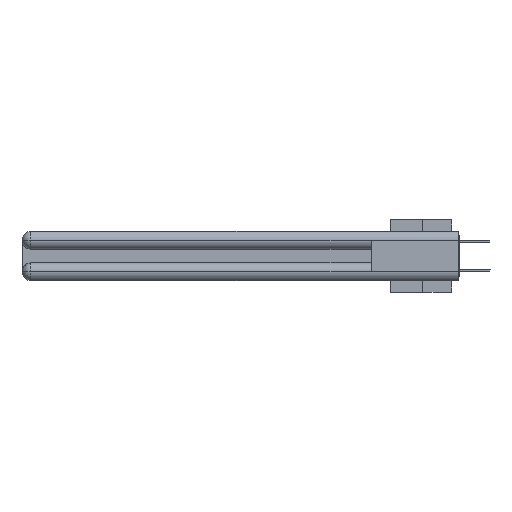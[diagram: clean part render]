
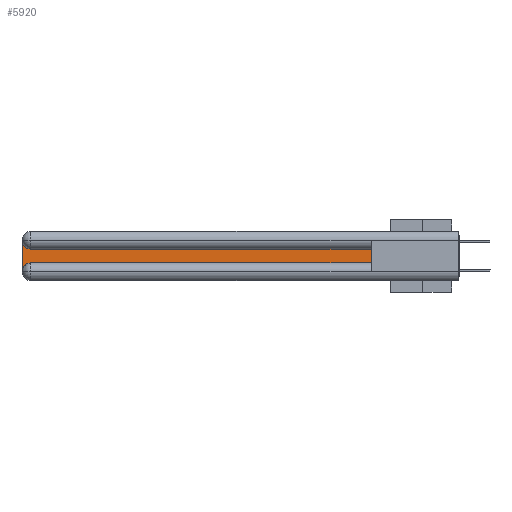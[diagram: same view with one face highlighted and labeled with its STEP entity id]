
A CAD part, left-side view. The second image highlights one B-rep face of the part: STEP entity #5920.
In plain terms, the highlighted planar face has unit normal (-1, 0, 0).
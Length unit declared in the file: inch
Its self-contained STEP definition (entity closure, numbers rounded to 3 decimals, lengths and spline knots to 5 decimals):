
#1481 = CARTESIAN_POINT ( 'NONE',  ( 0.075, 0.6, -0.2175 ) ) ;
#1792 = CARTESIAN_POINT ( 'NONE',  ( 0.075, 0.6, -0.2175 ) ) ;
#2102 = ORIENTED_EDGE ( 'NONE', *, *, #15685, .T. ) ;
#2731 = ORIENTED_EDGE ( 'NONE', *, *, #14628, .T. ) ;
#2751 = ORIENTED_EDGE ( 'NONE', *, *, #28958, .T. ) ;
#3888 = CARTESIAN_POINT ( 'NONE',  ( 0.075, 3., -0.2775 ) ) ;
#4295 = DIRECTION ( 'NONE',  ( 0., 0., 1. ) ) ;
#4319 = LINE ( 'NONE', #1481, #8653 ) ;
#4943 = CARTESIAN_POINT ( 'NONE',  ( 0.075, 2.94, -0.1225 ) ) ;
#5920 = ADVANCED_FACE ( 'NONE', ( #34883 ), #7283, .F. ) ;
#6153 = LINE ( 'NONE', #12125, #27566 ) ;
#7283 = PLANE ( 'NONE',  #14987 ) ;
#7659 = ORIENTED_EDGE ( 'NONE', *, *, #33788, .T. ) ;
#8567 = LINE ( 'NONE', #12396, #33830 ) ;
#8653 = VECTOR ( 'NONE', #4295, 39.37008 ) ;
#9470 = DIRECTION ( 'NONE',  ( 1., 0., 0. ) ) ;
#9493 = LINE ( 'NONE', #20822, #21748 ) ;
#10178 = DIRECTION ( 'NONE',  ( 0., -1., 0. ) ) ;
#11277 = ORIENTED_EDGE ( 'NONE', *, *, #23849, .T. ) ;
#11372 = EDGE_CURVE ( 'NONE', #14433, #11629, #6153, .T. ) ;
#11629 = VERTEX_POINT ( 'NONE', #3888 ) ;
#12125 = CARTESIAN_POINT ( 'NONE',  ( 0.075, 3., -0.2175 ) ) ;
#12335 = CARTESIAN_POINT ( 'NONE',  ( 0.075, 3., -0.0625 ) ) ;
#12396 = CARTESIAN_POINT ( 'NONE',  ( 0.075, 0.6, -0.1225 ) ) ;
#14433 = VERTEX_POINT ( 'NONE', #12335 ) ;
#14442 = VERTEX_POINT ( 'NONE', #32348 ) ;
#14628 = EDGE_CURVE ( 'NONE', #14442, #19472, #8567, .T. ) ;
#14987 = AXIS2_PLACEMENT_3D ( 'NONE', #15819, #24259, #35648 ) ;
#15364 = AXIS2_PLACEMENT_3D ( 'NONE', #23409, #9470, #26465 ) ;
#15685 = EDGE_CURVE ( 'NONE', #11629, #19381, #32975, .T. ) ;
#15819 = CARTESIAN_POINT ( 'NONE',  ( 0.075, 3., -0.1225 ) ) ;
#15835 = VERTEX_POINT ( 'NONE', #1792 ) ;
#16766 = CARTESIAN_POINT ( 'NONE',  ( 0.075, 2.94, -0.0625 ) ) ;
#17237 = DIRECTION ( 'NONE',  ( 1., 0., 0. ) ) ;
#19381 = VERTEX_POINT ( 'NONE', #26808 ) ;
#19472 = VERTEX_POINT ( 'NONE', #4943 ) ;
#19587 = DIRECTION ( 'NONE',  ( 0., 0., -1. ) ) ;
#20557 = DIRECTION ( 'NONE',  ( 0., 0., -1. ) ) ;
#20822 = CARTESIAN_POINT ( 'NONE',  ( 0.075, 0.6, -0.2175 ) ) ;
#21748 = VECTOR ( 'NONE', #10178, 39.37008 ) ;
#23409 = CARTESIAN_POINT ( 'NONE',  ( 0.075, 2.94, -0.2775 ) ) ;
#23521 = CIRCLE ( 'NONE', #31676, 0.06 ) ;
#23849 = EDGE_CURVE ( 'NONE', #19381, #15835, #9493, .T. ) ;
#24007 = DIRECTION ( 'NONE',  ( 0., 1., 0. ) ) ;
#24259 = DIRECTION ( 'NONE',  ( 1., 0., 0. ) ) ;
#24705 = ORIENTED_EDGE ( 'NONE', *, *, #11372, .T. ) ;
#26465 = DIRECTION ( 'NONE',  ( 0., 0., -1. ) ) ;
#26808 = CARTESIAN_POINT ( 'NONE',  ( 0.075, 2.94, -0.2175 ) ) ;
#27566 = VECTOR ( 'NONE', #20557, 39.37008 ) ;
#28958 = EDGE_CURVE ( 'NONE', #15835, #14442, #4319, .T. ) ;
#31676 = AXIS2_PLACEMENT_3D ( 'NONE', #16766, #17237, #19587 ) ;
#32348 = CARTESIAN_POINT ( 'NONE',  ( 0.075, 0.6, -0.1225 ) ) ;
#32903 = EDGE_LOOP ( 'NONE', ( #2731, #7659, #24705, #2102, #11277, #2751 ) ) ;
#32975 = CIRCLE ( 'NONE', #15364, 0.06 ) ;
#33788 = EDGE_CURVE ( 'NONE', #19472, #14433, #23521, .T. ) ;
#33830 = VECTOR ( 'NONE', #24007, 39.37008 ) ;
#34883 = FACE_OUTER_BOUND ( 'NONE', #32903, .T. ) ;
#35648 = DIRECTION ( 'NONE',  ( 0., 0., -1. ) ) ;
